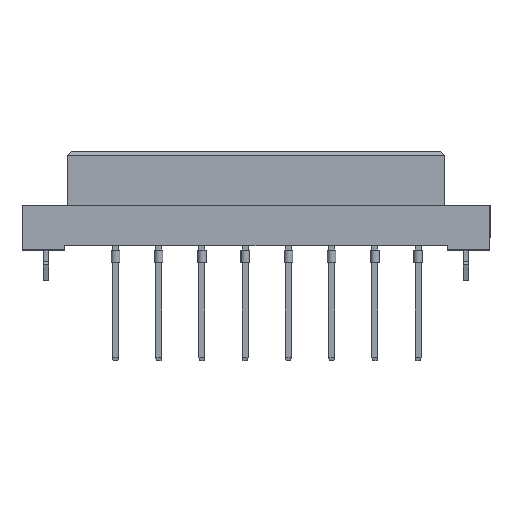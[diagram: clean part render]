
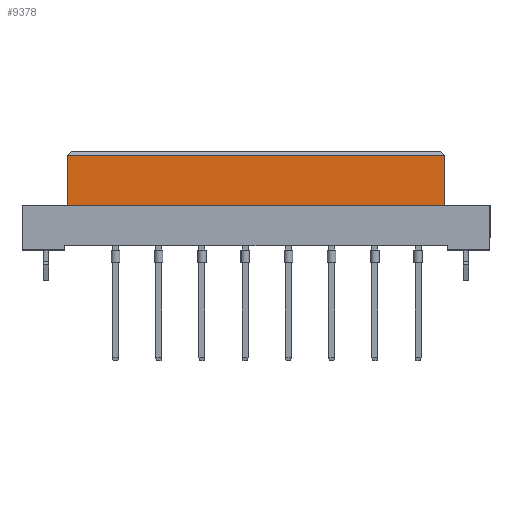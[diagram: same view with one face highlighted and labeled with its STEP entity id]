
A CAD part, top view. The second image highlights one B-rep face of the part: STEP entity #9378.
In plain terms, the highlighted planar face has unit normal (0, 0, 1).
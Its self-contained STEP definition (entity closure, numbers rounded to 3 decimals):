
#17 = VECTOR ( 'NONE', #271, 1000. ) ;
#180 = ORIENTED_EDGE ( 'NONE', *, *, #21432, .T. ) ;
#251 = EDGE_CURVE ( 'NONE', #12402, #7277, #565, .T. ) ;
#271 = DIRECTION ( 'NONE',  ( 1., 0., 0. ) ) ;
#388 = CARTESIAN_POINT ( 'NONE',  ( 22.2, -6.4, 4.25 ) ) ;
#565 = LINE ( 'NONE', #14042, #7925 ) ;
#1101 = CARTESIAN_POINT ( 'NONE',  ( -22.2, -0.5, 4.25 ) ) ;
#1485 = CARTESIAN_POINT ( 'NONE',  ( 22.2, -6.4, 4.25 ) ) ;
#1870 = VECTOR ( 'NONE', #15546, 1000. ) ;
#3416 = CARTESIAN_POINT ( 'NONE',  ( 22.2, -6.4, 4.25 ) ) ;
#3422 = VERTEX_POINT ( 'NONE', #5685 ) ;
#5685 = CARTESIAN_POINT ( 'NONE',  ( 22.2, -0.5, 4.25 ) ) ;
#6203 = CARTESIAN_POINT ( 'NONE',  ( -22.2, -6.4, 4.25 ) ) ;
#7277 = VERTEX_POINT ( 'NONE', #1101 ) ;
#7530 = EDGE_LOOP ( 'NONE', ( #180, #16042, #9668, #7884 ) ) ;
#7803 = EDGE_CURVE ( 'NONE', #12402, #11860, #8417, .T. ) ;
#7884 = ORIENTED_EDGE ( 'NONE', *, *, #7803, .T. ) ;
#7925 = VECTOR ( 'NONE', #18689, 1000. ) ;
#8417 = LINE ( 'NONE', #1485, #17 ) ;
#8610 = PLANE ( 'NONE',  #9008 ) ;
#9008 = AXIS2_PLACEMENT_3D ( 'NONE', #3416, #20032, #19720 ) ;
#9378 = ADVANCED_FACE ( 'NONE', ( #16881 ), #8610, .T. ) ;
#9668 = ORIENTED_EDGE ( 'NONE', *, *, #251, .F. ) ;
#9848 = CARTESIAN_POINT ( 'NONE',  ( 22.2, -6.4, 4.25 ) ) ;
#11860 = VERTEX_POINT ( 'NONE', #9848 ) ;
#12402 = VERTEX_POINT ( 'NONE', #6203 ) ;
#13935 = EDGE_CURVE ( 'NONE', #3422, #7277, #20122, .T. ) ;
#14023 = VECTOR ( 'NONE', #20472, 1000. ) ;
#14042 = CARTESIAN_POINT ( 'NONE',  ( -22.2, -6.4, 4.25 ) ) ;
#15546 = DIRECTION ( 'NONE',  ( -1., 0., 0. ) ) ;
#15575 = LINE ( 'NONE', #388, #14023 ) ;
#16042 = ORIENTED_EDGE ( 'NONE', *, *, #13935, .T. ) ;
#16866 = CARTESIAN_POINT ( 'NONE',  ( -22.2, -0.5, 4.25 ) ) ;
#16881 = FACE_OUTER_BOUND ( 'NONE', #7530, .T. ) ;
#18689 = DIRECTION ( 'NONE',  ( 0., 1., 0. ) ) ;
#19720 = DIRECTION ( 'NONE',  ( 1., 0., 0. ) ) ;
#20032 = DIRECTION ( 'NONE',  ( 0., 0., 1. ) ) ;
#20122 = LINE ( 'NONE', #16866, #1870 ) ;
#20472 = DIRECTION ( 'NONE',  ( 0., 1., 0. ) ) ;
#21432 = EDGE_CURVE ( 'NONE', #11860, #3422, #15575, .T. ) ;
